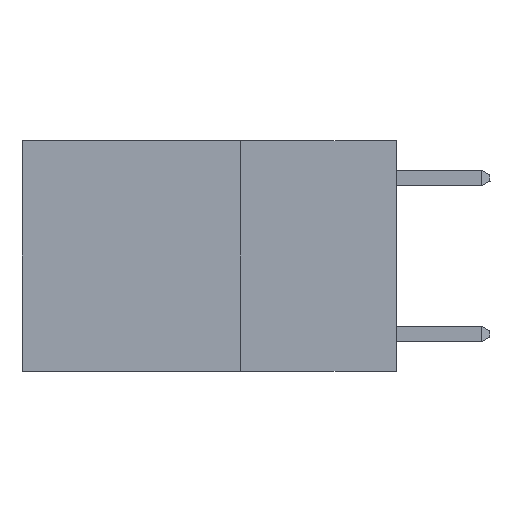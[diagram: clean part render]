
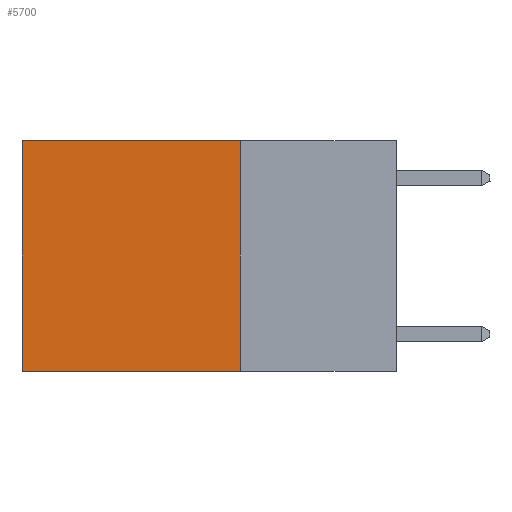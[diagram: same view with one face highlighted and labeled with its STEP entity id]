
A CAD part, left-side view. The second image highlights one B-rep face of the part: STEP entity #5700.
In plain terms, the highlighted planar face has unit normal (-1, 0, 0).
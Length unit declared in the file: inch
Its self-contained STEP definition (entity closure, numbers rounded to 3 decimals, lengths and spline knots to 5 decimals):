
#252 = CARTESIAN_POINT ( 'NONE',  ( 0.2625, 0.25, 0. ) ) ;
#370 = ORIENTED_EDGE ( 'NONE', *, *, #12372, .T. ) ;
#730 = DIRECTION ( 'NONE',  ( 0., 0., -1. ) ) ;
#1407 = CARTESIAN_POINT ( 'NONE',  ( 0.2625, 0.25, -0.37 ) ) ;
#1896 = LINE ( 'NONE', #6001, #12961 ) ;
#1963 = CARTESIAN_POINT ( 'NONE',  ( 0.2625, 0.6, 0. ) ) ;
#2023 = CARTESIAN_POINT ( 'NONE',  ( 0.2625, 0.25, 0. ) ) ;
#2191 = LINE ( 'NONE', #10052, #15033 ) ;
#2205 = VERTEX_POINT ( 'NONE', #1407 ) ;
#2284 = VERTEX_POINT ( 'NONE', #2952 ) ;
#2489 = EDGE_CURVE ( 'NONE', #14182, #2205, #13088, .T. ) ;
#2900 = LINE ( 'NONE', #10439, #15907 ) ;
#2952 = CARTESIAN_POINT ( 'NONE',  ( 0.2625, 0.6, -0.37 ) ) ;
#3864 = DIRECTION ( 'NONE',  ( 0., 0., -1. ) ) ;
#4731 = VERTEX_POINT ( 'NONE', #1963 ) ;
#4851 = ORIENTED_EDGE ( 'NONE', *, *, #2489, .F. ) ;
#5700 = ADVANCED_FACE ( 'NONE', ( #12004 ), #7620, .F. ) ;
#6001 = CARTESIAN_POINT ( 'NONE',  ( 0.2625, 0.25, 0. ) ) ;
#7620 = PLANE ( 'NONE',  #8559 ) ;
#8559 = AXIS2_PLACEMENT_3D ( 'NONE', #252, #10139, #730 ) ;
#8678 = EDGE_CURVE ( 'NONE', #2205, #2284, #2900, .T. ) ;
#8916 = DIRECTION ( 'NONE',  ( 0., 1., 0. ) ) ;
#9510 = DIRECTION ( 'NONE',  ( 0., 1., 0. ) ) ;
#9730 = EDGE_CURVE ( 'NONE', #14182, #4731, #1896, .T. ) ;
#10052 = CARTESIAN_POINT ( 'NONE',  ( 0.2625, 0.6, 0. ) ) ;
#10139 = DIRECTION ( 'NONE',  ( 1., 0., 0. ) ) ;
#10439 = CARTESIAN_POINT ( 'NONE',  ( 0.2625, 0.25, -0.37 ) ) ;
#11678 = ORIENTED_EDGE ( 'NONE', *, *, #8678, .F. ) ;
#12004 = FACE_OUTER_BOUND ( 'NONE', #14494, .T. ) ;
#12104 = VECTOR ( 'NONE', #15796, 39.37008 ) ;
#12372 = EDGE_CURVE ( 'NONE', #4731, #2284, #2191, .T. ) ;
#12961 = VECTOR ( 'NONE', #8916, 39.37008 ) ;
#13088 = LINE ( 'NONE', #2023, #12104 ) ;
#14182 = VERTEX_POINT ( 'NONE', #15364 ) ;
#14494 = EDGE_LOOP ( 'NONE', ( #370, #11678, #4851, #16000 ) ) ;
#15033 = VECTOR ( 'NONE', #3864, 39.37008 ) ;
#15364 = CARTESIAN_POINT ( 'NONE',  ( 0.2625, 0.25, 0. ) ) ;
#15796 = DIRECTION ( 'NONE',  ( 0., 0., -1. ) ) ;
#15907 = VECTOR ( 'NONE', #9510, 39.37008 ) ;
#16000 = ORIENTED_EDGE ( 'NONE', *, *, #9730, .T. ) ;
